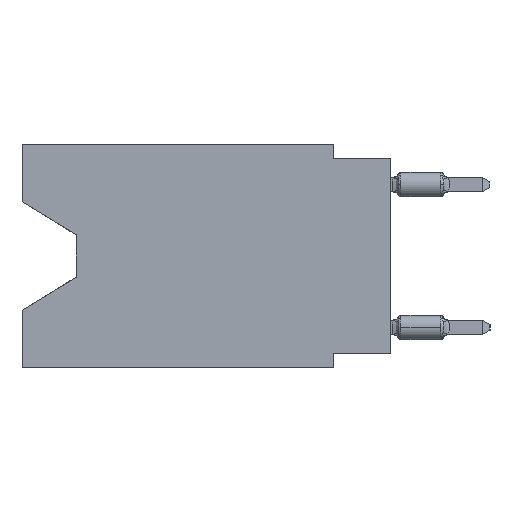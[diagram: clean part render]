
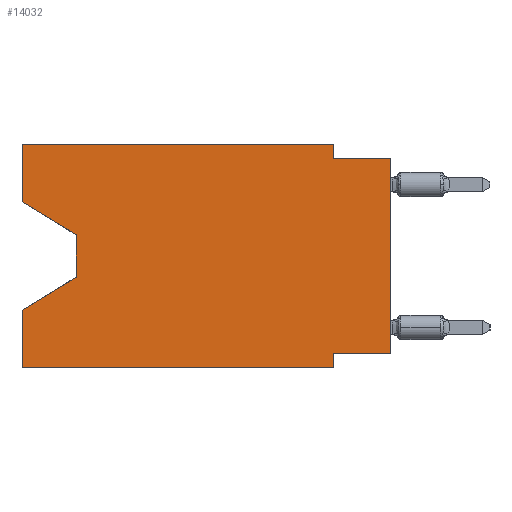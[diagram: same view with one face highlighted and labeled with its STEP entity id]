
A CAD part, left-side view. The second image highlights one B-rep face of the part: STEP entity #14032.
In plain terms, the highlighted planar face has unit normal (-1, 0, 0).
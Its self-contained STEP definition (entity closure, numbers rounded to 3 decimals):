
#464 = EDGE_CURVE ( 'NONE', #21589, #21208, #11294, .T. ) ;
#1096 = CARTESIAN_POINT ( 'NONE',  ( 0., 0., -0.635 ) ) ;
#2097 = CARTESIAN_POINT ( 'NONE',  ( 0., 16.383, 0. ) ) ;
#2284 = CARTESIAN_POINT ( 'NONE',  ( 0., 16.383, -2.546 ) ) ;
#2774 = VECTOR ( 'NONE', #7883, 1000. ) ;
#3320 = VERTEX_POINT ( 'NONE', #39467 ) ;
#3801 = VERTEX_POINT ( 'NONE', #28885 ) ;
#4027 = VECTOR ( 'NONE', #6536, 1000. ) ;
#4172 = VERTEX_POINT ( 'NONE', #12108 ) ;
#4360 = DIRECTION ( 'NONE',  ( 0., 0., -1. ) ) ;
#5103 = CARTESIAN_POINT ( 'NONE',  ( 0., 13.97, -4.013 ) ) ;
#5288 = DIRECTION ( 'NONE',  ( 0., 0., 1. ) ) ;
#5298 = ORIENTED_EDGE ( 'NONE', *, *, #35043, .T. ) ;
#6268 = CARTESIAN_POINT ( 'NONE',  ( 0., 16.383, 0. ) ) ;
#6536 = DIRECTION ( 'NONE',  ( 0., -0.855, -0.519 ) ) ;
#7178 = ORIENTED_EDGE ( 'NONE', *, *, #42910, .F. ) ;
#7831 = EDGE_CURVE ( 'NONE', #21589, #30118, #35281, .T. ) ;
#7883 = DIRECTION ( 'NONE',  ( 0., -1., 0. ) ) ;
#8626 = VECTOR ( 'NONE', #21844, 1000. ) ;
#10339 = CARTESIAN_POINT ( 'NONE',  ( 0., 0., -0.635 ) ) ;
#10737 = VECTOR ( 'NONE', #21729, 1000. ) ;
#11105 = LINE ( 'NONE', #26357, #28853 ) ;
#11294 = LINE ( 'NONE', #26543, #42415 ) ;
#11631 = VERTEX_POINT ( 'NONE', #39000 ) ;
#11762 = VERTEX_POINT ( 'NONE', #31275 ) ;
#12108 = CARTESIAN_POINT ( 'NONE',  ( 0., 2.54, -9.906 ) ) ;
#12232 = EDGE_CURVE ( 'NONE', #3320, #42284, #37340, .T. ) ;
#13287 = EDGE_CURVE ( 'NONE', #21208, #4172, #34233, .T. ) ;
#14032 = ADVANCED_FACE ( 'NONE', ( #21146 ), #40602, .F. ) ;
#14130 = ORIENTED_EDGE ( 'NONE', *, *, #39069, .F. ) ;
#16578 = LINE ( 'NONE', #6268, #33297 ) ;
#16629 = CARTESIAN_POINT ( 'NONE',  ( 0., 2.54, 0. ) ) ;
#17854 = CARTESIAN_POINT ( 'NONE',  ( 0., 16.383, 0. ) ) ;
#18267 = VECTOR ( 'NONE', #34927, 1000. ) ;
#18335 = AXIS2_PLACEMENT_3D ( 'NONE', #2097, #47846, #25135 ) ;
#20573 = CARTESIAN_POINT ( 'NONE',  ( 0., 2.54, -9.271 ) ) ;
#20767 = CARTESIAN_POINT ( 'NONE',  ( 0., 2.54, 0. ) ) ;
#20783 = VECTOR ( 'NONE', #4360, 1000. ) ;
#20945 = CARTESIAN_POINT ( 'NONE',  ( 0., 16.383, 0. ) ) ;
#21008 = LINE ( 'NONE', #25002, #10737 ) ;
#21146 = FACE_OUTER_BOUND ( 'NONE', #46890, .T. ) ;
#21208 = VERTEX_POINT ( 'NONE', #20573 ) ;
#21589 = VERTEX_POINT ( 'NONE', #34777 ) ;
#21729 = DIRECTION ( 'NONE',  ( 0., -1., 0. ) ) ;
#21844 = DIRECTION ( 'NONE',  ( 0., -1., 0. ) ) ;
#22973 = EDGE_CURVE ( 'NONE', #3801, #4172, #21008, .T. ) ;
#23752 = EDGE_CURVE ( 'NONE', #11631, #42743, #11105, .T. ) ;
#25002 = CARTESIAN_POINT ( 'NONE',  ( 0., 16.383, -9.906 ) ) ;
#25135 = DIRECTION ( 'NONE',  ( 0., 0., -1. ) ) ;
#25166 = EDGE_CURVE ( 'NONE', #3320, #30927, #32335, .T. ) ;
#25685 = ORIENTED_EDGE ( 'NONE', *, *, #23752, .T. ) ;
#26309 = VECTOR ( 'NONE', #30351, 1000. ) ;
#26357 = CARTESIAN_POINT ( 'NONE',  ( 0., 13.97, -5.893 ) ) ;
#26543 = CARTESIAN_POINT ( 'NONE',  ( 0., 0., -9.271 ) ) ;
#26797 = ORIENTED_EDGE ( 'NONE', *, *, #464, .F. ) ;
#26908 = VECTOR ( 'NONE', #46750, 1000. ) ;
#27277 = DIRECTION ( 'NONE',  ( 0., 1., 0. ) ) ;
#27530 = CARTESIAN_POINT ( 'NONE',  ( 0., 0., 0. ) ) ;
#28108 = LINE ( 'NONE', #16629, #20783 ) ;
#28853 = VECTOR ( 'NONE', #41590, 1000. ) ;
#28885 = CARTESIAN_POINT ( 'NONE',  ( 0., 16.383, -9.906 ) ) ;
#29910 = CARTESIAN_POINT ( 'NONE',  ( 0., 13.97, -4.013 ) ) ;
#30118 = VERTEX_POINT ( 'NONE', #10339 ) ;
#30351 = DIRECTION ( 'NONE',  ( 0., 0., 1. ) ) ;
#30604 = CARTESIAN_POINT ( 'NONE',  ( 0., 16.383, 0. ) ) ;
#30927 = VERTEX_POINT ( 'NONE', #29910 ) ;
#31203 = ORIENTED_EDGE ( 'NONE', *, *, #12232, .F. ) ;
#31275 = CARTESIAN_POINT ( 'NONE',  ( 0., 2.54, -0.635 ) ) ;
#32335 = LINE ( 'NONE', #2284, #4027 ) ;
#33297 = VECTOR ( 'NONE', #5288, 1000. ) ;
#34233 = LINE ( 'NONE', #38717, #18267 ) ;
#34777 = CARTESIAN_POINT ( 'NONE',  ( 0., 0., -9.271 ) ) ;
#34927 = DIRECTION ( 'NONE',  ( 0., 0., -1. ) ) ;
#35043 = EDGE_CURVE ( 'NONE', #30927, #11631, #39369, .T. ) ;
#35281 = LINE ( 'NONE', #27530, #26908 ) ;
#35378 = EDGE_CURVE ( 'NONE', #11762, #30118, #42613, .T. ) ;
#36144 = ORIENTED_EDGE ( 'NONE', *, *, #37086, .F. ) ;
#36244 = ORIENTED_EDGE ( 'NONE', *, *, #22973, .T. ) ;
#37025 = ORIENTED_EDGE ( 'NONE', *, *, #25166, .T. ) ;
#37086 = EDGE_CURVE ( 'NONE', #3801, #42743, #16578, .T. ) ;
#37340 = LINE ( 'NONE', #20945, #26309 ) ;
#37343 = ORIENTED_EDGE ( 'NONE', *, *, #13287, .F. ) ;
#38717 = CARTESIAN_POINT ( 'NONE',  ( 0., 2.54, -9.906 ) ) ;
#39000 = CARTESIAN_POINT ( 'NONE',  ( 0., 13.97, -5.893 ) ) ;
#39069 = EDGE_CURVE ( 'NONE', #42284, #41119, #44330, .T. ) ;
#39369 = LINE ( 'NONE', #5103, #47462 ) ;
#39467 = CARTESIAN_POINT ( 'NONE',  ( 0., 16.383, -2.546 ) ) ;
#40602 = PLANE ( 'NONE',  #18335 ) ;
#41119 = VERTEX_POINT ( 'NONE', #20767 ) ;
#41590 = DIRECTION ( 'NONE',  ( 0., 0.855, -0.519 ) ) ;
#42284 = VERTEX_POINT ( 'NONE', #30604 ) ;
#42415 = VECTOR ( 'NONE', #27277, 1000. ) ;
#42613 = LINE ( 'NONE', #1096, #2774 ) ;
#42743 = VERTEX_POINT ( 'NONE', #47422 ) ;
#42910 = EDGE_CURVE ( 'NONE', #41119, #11762, #28108, .T. ) ;
#43351 = DIRECTION ( 'NONE',  ( 0., 0., -1. ) ) ;
#44330 = LINE ( 'NONE', #17854, #8626 ) ;
#45543 = ORIENTED_EDGE ( 'NONE', *, *, #7831, .T. ) ;
#46750 = DIRECTION ( 'NONE',  ( 0., 0., 1. ) ) ;
#46890 = EDGE_LOOP ( 'NONE', ( #37025, #5298, #25685, #36144, #36244, #37343, #26797, #45543, #48897, #7178, #14130, #31203 ) ) ;
#47422 = CARTESIAN_POINT ( 'NONE',  ( 0., 16.383, -7.36 ) ) ;
#47462 = VECTOR ( 'NONE', #43351, 1000. ) ;
#47846 = DIRECTION ( 'NONE',  ( 1., 0., 0. ) ) ;
#48897 = ORIENTED_EDGE ( 'NONE', *, *, #35378, .F. ) ;
